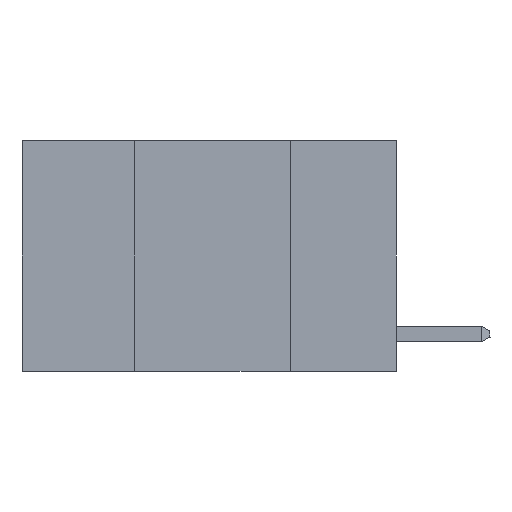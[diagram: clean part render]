
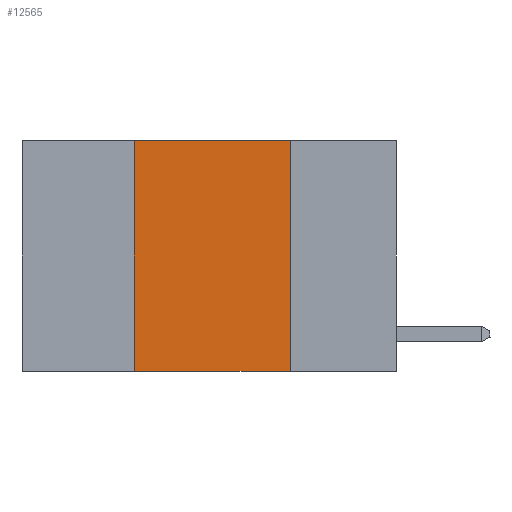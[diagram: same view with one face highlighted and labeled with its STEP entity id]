
A CAD part, left-side view. The second image highlights one B-rep face of the part: STEP entity #12565.
In plain terms, the highlighted planar face has unit normal (-1, 0, 0).
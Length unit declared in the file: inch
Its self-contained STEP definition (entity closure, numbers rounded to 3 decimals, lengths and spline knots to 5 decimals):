
#84 = CARTESIAN_POINT ( 'NONE',  ( 0., 0.6, 0. ) ) ;
#267 = VECTOR ( 'NONE', #13337, 39.37008 ) ;
#451 = DIRECTION ( 'NONE',  ( 0., -1., 0. ) ) ;
#1244 = VERTEX_POINT ( 'NONE', #6703 ) ;
#1251 = EDGE_CURVE ( 'NONE', #4223, #15771, #17575, .T. ) ;
#1764 = VERTEX_POINT ( 'NONE', #5404 ) ;
#1945 = EDGE_CURVE ( 'NONE', #1764, #1244, #16864, .T. ) ;
#2316 = FACE_OUTER_BOUND ( 'NONE', #3428, .T. ) ;
#2806 = ORIENTED_EDGE ( 'NONE', *, *, #7145, .F. ) ;
#3045 = CARTESIAN_POINT ( 'NONE',  ( 0., 0.17, 0. ) ) ;
#3428 = EDGE_LOOP ( 'NONE', ( #2806, #14592, #4791, #9002 ) ) ;
#4075 = LINE ( 'NONE', #11902, #267 ) ;
#4092 = CARTESIAN_POINT ( 'NONE',  ( 0., 0.6, 0. ) ) ;
#4223 = VERTEX_POINT ( 'NONE', #15933 ) ;
#4791 = ORIENTED_EDGE ( 'NONE', *, *, #17064, .F. ) ;
#5404 = CARTESIAN_POINT ( 'NONE',  ( 0., 0.42, 0. ) ) ;
#5544 = DIRECTION ( 'NONE',  ( 0., 0., -1. ) ) ;
#6703 = CARTESIAN_POINT ( 'NONE',  ( 0., 0.17, 0. ) ) ;
#7145 = EDGE_CURVE ( 'NONE', #1244, #15771, #16194, .T. ) ;
#9002 = ORIENTED_EDGE ( 'NONE', *, *, #1251, .T. ) ;
#9087 = VECTOR ( 'NONE', #10121, 39.37008 ) ;
#9211 = CARTESIAN_POINT ( 'NONE',  ( 0., 0.6, -0.37 ) ) ;
#9303 = VECTOR ( 'NONE', #451, 39.37008 ) ;
#10121 = DIRECTION ( 'NONE',  ( 0., 0., -1. ) ) ;
#11156 = PLANE ( 'NONE',  #11686 ) ;
#11686 = AXIS2_PLACEMENT_3D ( 'NONE', #4092, #14042, #5544 ) ;
#11902 = CARTESIAN_POINT ( 'NONE',  ( 0., 0.42, 0. ) ) ;
#12067 = CARTESIAN_POINT ( 'NONE',  ( 0., 0.17, -0.37 ) ) ;
#12565 = ADVANCED_FACE ( 'NONE', ( #2316 ), #11156, .F. ) ;
#13337 = DIRECTION ( 'NONE',  ( 0., 0., 1. ) ) ;
#13772 = VECTOR ( 'NONE', #16163, 39.37008 ) ;
#14042 = DIRECTION ( 'NONE',  ( 1., 0., 0. ) ) ;
#14592 = ORIENTED_EDGE ( 'NONE', *, *, #1945, .F. ) ;
#15771 = VERTEX_POINT ( 'NONE', #12067 ) ;
#15933 = CARTESIAN_POINT ( 'NONE',  ( 0., 0.42, -0.37 ) ) ;
#16163 = DIRECTION ( 'NONE',  ( 0., -1., 0. ) ) ;
#16194 = LINE ( 'NONE', #3045, #9087 ) ;
#16864 = LINE ( 'NONE', #84, #9303 ) ;
#17064 = EDGE_CURVE ( 'NONE', #4223, #1764, #4075, .T. ) ;
#17575 = LINE ( 'NONE', #9211, #13772 ) ;
